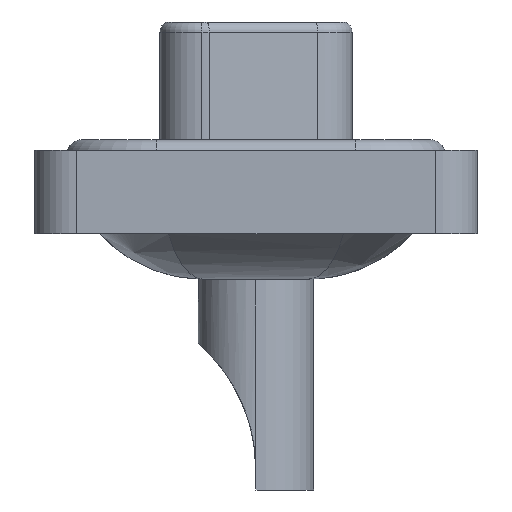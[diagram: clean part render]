
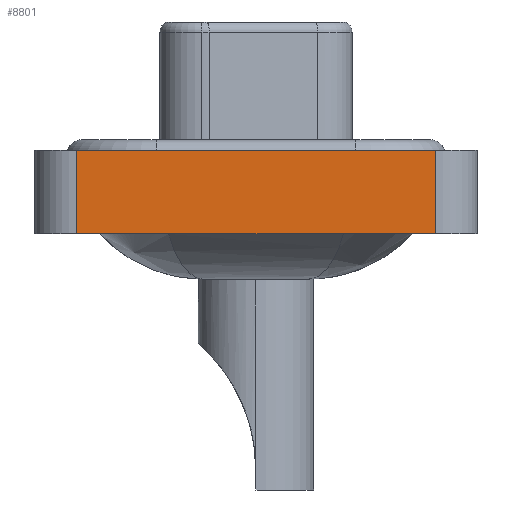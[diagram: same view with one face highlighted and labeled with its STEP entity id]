
A CAD part, left-side view. The second image highlights one B-rep face of the part: STEP entity #8801.
In plain terms, the highlighted planar face has unit normal (-1, 0, 0).
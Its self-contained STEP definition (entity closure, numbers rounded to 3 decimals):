
#236 = DIRECTION ( 'NONE',  ( -1., 0., 0. ) ) ;
#745 = DIRECTION ( 'NONE',  ( 0., -1., 0. ) ) ;
#934 = EDGE_CURVE ( 'NONE', #8134, #5304, #11477, .T. ) ;
#1242 = PLANE ( 'NONE',  #16154 ) ;
#1402 = FACE_OUTER_BOUND ( 'NONE', #12040, .T. ) ;
#1530 = ORIENTED_EDGE ( 'NONE', *, *, #934, .T. ) ;
#1601 = ORIENTED_EDGE ( 'NONE', *, *, #8574, .F. ) ;
#3566 = DIRECTION ( 'NONE',  ( 0., 0., 1. ) ) ;
#3745 = VECTOR ( 'NONE', #9119, 1000. ) ;
#4359 = VECTOR ( 'NONE', #745, 1000. ) ;
#5092 = CARTESIAN_POINT ( 'NONE',  ( -7.3, -8.55, -3.6 ) ) ;
#5105 = CARTESIAN_POINT ( 'NONE',  ( -7.3, -8.55, 0.4 ) ) ;
#5109 = CARTESIAN_POINT ( 'NONE',  ( -7.3, 8.55, -3.6 ) ) ;
#5263 = DIRECTION ( 'NONE',  ( 0., 0., 1. ) ) ;
#5304 = VERTEX_POINT ( 'NONE', #14009 ) ;
#5955 = ORIENTED_EDGE ( 'NONE', *, *, #10310, .T. ) ;
#7192 = ORIENTED_EDGE ( 'NONE', *, *, #9504, .F. ) ;
#7404 = LINE ( 'NONE', #16324, #15644 ) ;
#7525 = CARTESIAN_POINT ( 'NONE',  ( -7.3, 8.55, -3.6 ) ) ;
#7765 = CARTESIAN_POINT ( 'NONE',  ( -7.3, -8.55, -3.6 ) ) ;
#7876 = VERTEX_POINT ( 'NONE', #5105 ) ;
#8134 = VERTEX_POINT ( 'NONE', #7525 ) ;
#8574 = EDGE_CURVE ( 'NONE', #16491, #7876, #12238, .T. ) ;
#8605 = CARTESIAN_POINT ( 'NONE',  ( -7.3, -8.55, 0.4 ) ) ;
#8801 = ADVANCED_FACE ( 'NONE', ( #1402 ), #1242, .T. ) ;
#8936 = VECTOR ( 'NONE', #12752, 1000. ) ;
#9119 = DIRECTION ( 'NONE',  ( 0., -1., 0. ) ) ;
#9504 = EDGE_CURVE ( 'NONE', #8134, #16491, #10483, .T. ) ;
#10310 = EDGE_CURVE ( 'NONE', #5304, #7876, #7404, .T. ) ;
#10483 = LINE ( 'NONE', #5109, #8936 ) ;
#11477 = LINE ( 'NONE', #5092, #3745 ) ;
#12040 = EDGE_LOOP ( 'NONE', ( #5955, #1601, #7192, #1530 ) ) ;
#12238 = LINE ( 'NONE', #8605, #4359 ) ;
#12752 = DIRECTION ( 'NONE',  ( 0., 0., 1. ) ) ;
#13264 = CARTESIAN_POINT ( 'NONE',  ( -7.3, 8.55, 0.4 ) ) ;
#14009 = CARTESIAN_POINT ( 'NONE',  ( -7.3, -8.55, -3.6 ) ) ;
#15644 = VECTOR ( 'NONE', #3566, 1000. ) ;
#16154 = AXIS2_PLACEMENT_3D ( 'NONE', #7765, #236, #5263 ) ;
#16324 = CARTESIAN_POINT ( 'NONE',  ( -7.3, -8.55, -3.6 ) ) ;
#16491 = VERTEX_POINT ( 'NONE', #13264 ) ;
